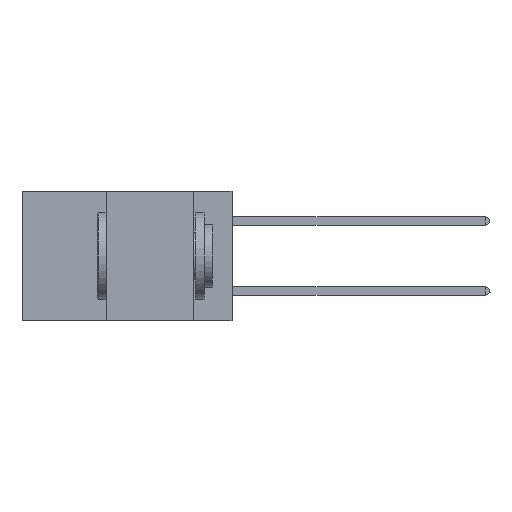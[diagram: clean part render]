
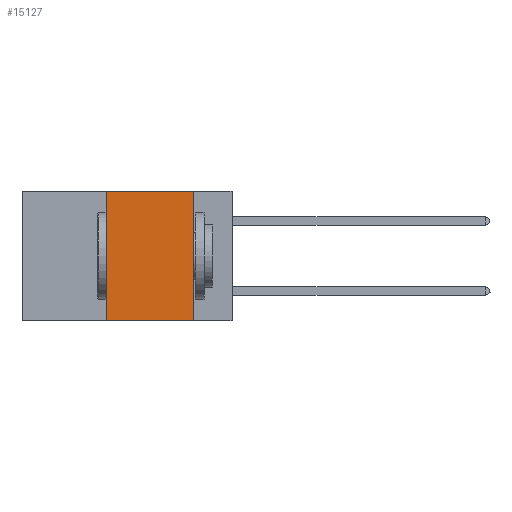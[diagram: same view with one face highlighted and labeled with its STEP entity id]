
A CAD part, left-side view. The second image highlights one B-rep face of the part: STEP entity #15127.
In plain terms, the highlighted planar face has unit normal (-1, 0, 0).
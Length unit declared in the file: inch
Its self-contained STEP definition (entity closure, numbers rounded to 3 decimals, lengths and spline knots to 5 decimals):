
#285 = CARTESIAN_POINT ( 'NONE',  ( 0., 0.6, 0. ) ) ;
#403 = EDGE_CURVE ( 'NONE', #5172, #13417, #4980, .T. ) ;
#806 = CARTESIAN_POINT ( 'NONE',  ( 0., 0.36, 0. ) ) ;
#932 = DIRECTION ( 'NONE',  ( 0., 0., -1. ) ) ;
#1200 = EDGE_CURVE ( 'NONE', #17179, #5172, #4687, .T. ) ;
#1345 = LINE ( 'NONE', #11318, #12076 ) ;
#1989 = VECTOR ( 'NONE', #15934, 39.37008 ) ;
#3593 = EDGE_CURVE ( 'NONE', #20757, #17179, #1345, .T. ) ;
#3716 = PLANE ( 'NONE',  #19098 ) ;
#4687 = LINE ( 'NONE', #18246, #21698 ) ;
#4980 = LINE ( 'NONE', #14571, #6335 ) ;
#5172 = VERTEX_POINT ( 'NONE', #21534 ) ;
#5783 = FACE_OUTER_BOUND ( 'NONE', #9262, .T. ) ;
#5801 = ORIENTED_EDGE ( 'NONE', *, *, #1200, .F. ) ;
#6007 = CARTESIAN_POINT ( 'NONE',  ( 0., 0.6, -0.37 ) ) ;
#6335 = VECTOR ( 'NONE', #16350, 39.37008 ) ;
#7698 = CARTESIAN_POINT ( 'NONE',  ( 0., 0.36, -0.37 ) ) ;
#7991 = DIRECTION ( 'NONE',  ( 0., 0., 1. ) ) ;
#9262 = EDGE_LOOP ( 'NONE', ( #10921, #5801, #9896, #16430 ) ) ;
#9896 = ORIENTED_EDGE ( 'NONE', *, *, #3593, .F. ) ;
#10921 = ORIENTED_EDGE ( 'NONE', *, *, #403, .F. ) ;
#11318 = CARTESIAN_POINT ( 'NONE',  ( 0., 0.36, 0. ) ) ;
#12076 = VECTOR ( 'NONE', #7991, 39.37008 ) ;
#12123 = CARTESIAN_POINT ( 'NONE',  ( 0., 0.11, -0.37 ) ) ;
#13417 = VERTEX_POINT ( 'NONE', #12123 ) ;
#14571 = CARTESIAN_POINT ( 'NONE',  ( 0., 0.11, 0. ) ) ;
#15127 = ADVANCED_FACE ( 'NONE', ( #5783 ), #3716, .F. ) ;
#15934 = DIRECTION ( 'NONE',  ( 0., -1., 0. ) ) ;
#16350 = DIRECTION ( 'NONE',  ( 0., 0., -1. ) ) ;
#16430 = ORIENTED_EDGE ( 'NONE', *, *, #17056, .T. ) ;
#17056 = EDGE_CURVE ( 'NONE', #20757, #13417, #17974, .T. ) ;
#17179 = VERTEX_POINT ( 'NONE', #806 ) ;
#17974 = LINE ( 'NONE', #6007, #1989 ) ;
#18246 = CARTESIAN_POINT ( 'NONE',  ( 0., 0.6, 0. ) ) ;
#19098 = AXIS2_PLACEMENT_3D ( 'NONE', #285, #21414, #932 ) ;
#19653 = DIRECTION ( 'NONE',  ( 0., -1., 0. ) ) ;
#20757 = VERTEX_POINT ( 'NONE', #7698 ) ;
#21414 = DIRECTION ( 'NONE',  ( 1., 0., 0. ) ) ;
#21534 = CARTESIAN_POINT ( 'NONE',  ( 0., 0.11, 0. ) ) ;
#21698 = VECTOR ( 'NONE', #19653, 39.37008 ) ;
